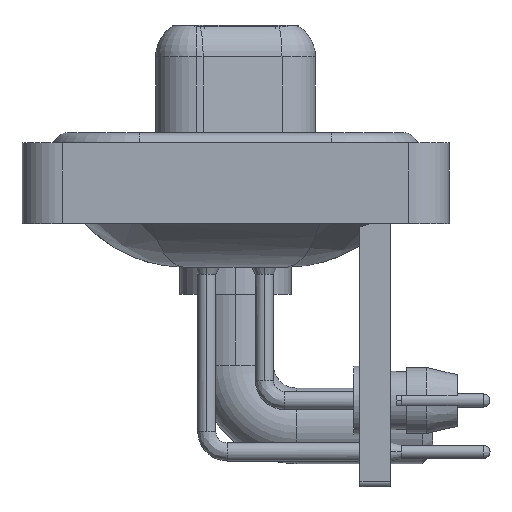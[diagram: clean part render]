
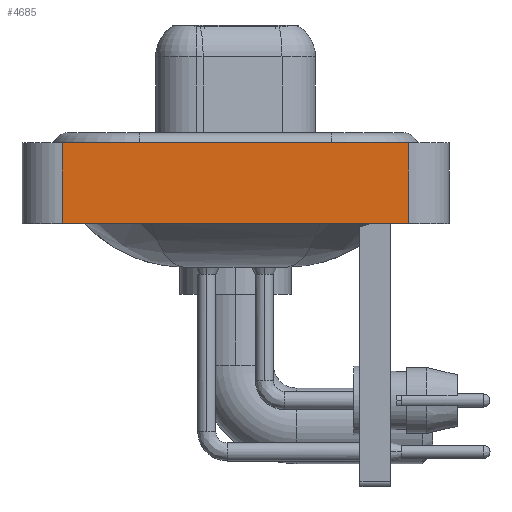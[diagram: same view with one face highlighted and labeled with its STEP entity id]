
A CAD part, left-side view. The second image highlights one B-rep face of the part: STEP entity #4685.
In plain terms, the highlighted planar face has unit normal (-1, 0, 0).
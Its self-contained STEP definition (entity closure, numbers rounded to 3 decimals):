
#247 = DIRECTION ( 'NONE',  ( 0., 0., 1. ) ) ;
#2828 = DIRECTION ( 'NONE',  ( 0., 0., 1. ) ) ;
#2900 = EDGE_CURVE ( 'NONE', #18659, #6174, #3207, .T. ) ;
#3163 = ORIENTED_EDGE ( 'NONE', *, *, #15200, .T. ) ;
#3207 = LINE ( 'NONE', #18466, #14358 ) ;
#3224 = VECTOR ( 'NONE', #20915, 1000. ) ;
#3810 = VECTOR ( 'NONE', #247, 1000. ) ;
#4157 = FACE_OUTER_BOUND ( 'NONE', #5260, .T. ) ;
#4493 = PLANE ( 'NONE',  #5038 ) ;
#4611 = CARTESIAN_POINT ( 'NONE',  ( -7.25, -8.55, -3.6 ) ) ;
#4685 = ADVANCED_FACE ( 'NONE', ( #4157 ), #4493, .T. ) ;
#4996 = CARTESIAN_POINT ( 'NONE',  ( -7.25, -8.55, 0.4 ) ) ;
#5038 = AXIS2_PLACEMENT_3D ( 'NONE', #4611, #13181, #2828 ) ;
#5260 = EDGE_LOOP ( 'NONE', ( #3163, #10739, #10663, #9511 ) ) ;
#5430 = VERTEX_POINT ( 'NONE', #15865 ) ;
#6174 = VERTEX_POINT ( 'NONE', #6632 ) ;
#6632 = CARTESIAN_POINT ( 'NONE',  ( -7.25, -8.55, -3.6 ) ) ;
#7245 = LINE ( 'NONE', #17533, #3810 ) ;
#8413 = VERTEX_POINT ( 'NONE', #4996 ) ;
#8882 = LINE ( 'NONE', #21243, #3224 ) ;
#9511 = ORIENTED_EDGE ( 'NONE', *, *, #2900, .T. ) ;
#9515 = EDGE_CURVE ( 'NONE', #18659, #5430, #7245, .T. ) ;
#9530 = CARTESIAN_POINT ( 'NONE',  ( -7.25, -8.55, -3.6 ) ) ;
#10013 = CARTESIAN_POINT ( 'NONE',  ( -7.25, 8.55, -3.6 ) ) ;
#10222 = VECTOR ( 'NONE', #14641, 1000. ) ;
#10663 = ORIENTED_EDGE ( 'NONE', *, *, #9515, .F. ) ;
#10739 = ORIENTED_EDGE ( 'NONE', *, *, #20301, .F. ) ;
#13181 = DIRECTION ( 'NONE',  ( -1., 0., 0. ) ) ;
#14358 = VECTOR ( 'NONE', #16763, 1000. ) ;
#14526 = LINE ( 'NONE', #9530, #10222 ) ;
#14641 = DIRECTION ( 'NONE',  ( 0., 0., 1. ) ) ;
#15200 = EDGE_CURVE ( 'NONE', #6174, #8413, #14526, .T. ) ;
#15865 = CARTESIAN_POINT ( 'NONE',  ( -7.25, 8.55, 0.4 ) ) ;
#16763 = DIRECTION ( 'NONE',  ( 0., -1., 0. ) ) ;
#17533 = CARTESIAN_POINT ( 'NONE',  ( -7.25, 8.55, -3.6 ) ) ;
#18466 = CARTESIAN_POINT ( 'NONE',  ( -7.25, -8.55, -3.6 ) ) ;
#18659 = VERTEX_POINT ( 'NONE', #10013 ) ;
#20301 = EDGE_CURVE ( 'NONE', #5430, #8413, #8882, .T. ) ;
#20915 = DIRECTION ( 'NONE',  ( 0., -1., 0. ) ) ;
#21243 = CARTESIAN_POINT ( 'NONE',  ( -7.25, -8.55, 0.4 ) ) ;
